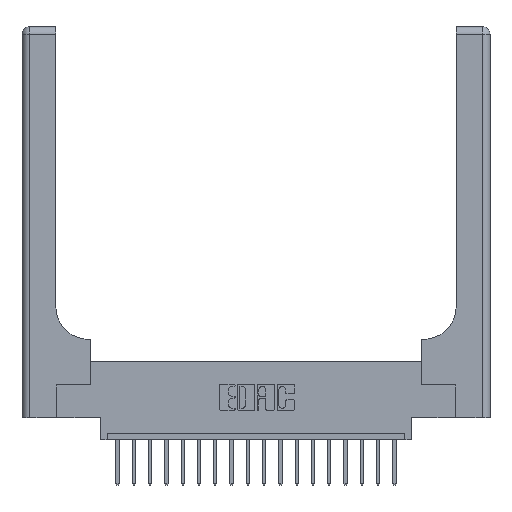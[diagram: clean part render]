
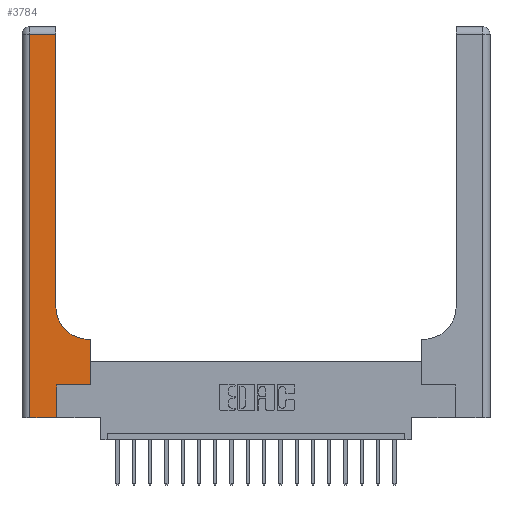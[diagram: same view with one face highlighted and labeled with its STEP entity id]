
A CAD part, top view. The second image highlights one B-rep face of the part: STEP entity #3784.
In plain terms, the highlighted planar face has unit normal (0, 0, 1).
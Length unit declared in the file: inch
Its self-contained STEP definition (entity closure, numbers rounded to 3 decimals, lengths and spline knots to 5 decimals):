
#433 = EDGE_CURVE ( 'NONE', #9430, #5543, #11502, .T. ) ;
#512 = VERTEX_POINT ( 'NONE', #19028 ) ;
#1346 = CARTESIAN_POINT ( 'NONE',  ( 0.26, 2.94, 0.37 ) ) ;
#1496 = PLANE ( 'NONE',  #4193 ) ;
#1530 = ORIENTED_EDGE ( 'NONE', *, *, #11882, .T. ) ;
#1644 = CARTESIAN_POINT ( 'NONE',  ( 0.528, 0.6, 0.37 ) ) ;
#1935 = EDGE_CURVE ( 'NONE', #7485, #10852, #15065, .T. ) ;
#1997 = DIRECTION ( 'NONE',  ( -1., 0., 0. ) ) ;
#2199 = EDGE_CURVE ( 'NONE', #10852, #9343, #11378, .T. ) ;
#2206 = CARTESIAN_POINT ( 'NONE',  ( 0.06, 3., 0.37 ) ) ;
#2723 = CARTESIAN_POINT ( 'NONE',  ( 0.26, 3., 0.37 ) ) ;
#2942 = CIRCLE ( 'NONE', #10118, 0.25 ) ;
#3034 = DIRECTION ( 'NONE',  ( 0., 0., -1. ) ) ;
#3057 = CARTESIAN_POINT ( 'NONE',  ( 0.265, 0., 0.37 ) ) ;
#3190 = ORIENTED_EDGE ( 'NONE', *, *, #14897, .T. ) ;
#3748 = DIRECTION ( 'NONE',  ( 0., 0., -1. ) ) ;
#3783 = EDGE_LOOP ( 'NONE', ( #17732, #6560, #5774, #9302, #17265, #17860, #12624, #1530, #3190 ) ) ;
#3784 = ADVANCED_FACE ( 'NONE', ( #13866 ), #1496, .F. ) ;
#4193 = AXIS2_PLACEMENT_3D ( 'NONE', #4578, #3034, #12538 ) ;
#4578 = CARTESIAN_POINT ( 'NONE',  ( 0., 3., 0.37 ) ) ;
#4712 = VERTEX_POINT ( 'NONE', #10948 ) ;
#5342 = DIRECTION ( 'NONE',  ( 0., 1., 0. ) ) ;
#5543 = VERTEX_POINT ( 'NONE', #14847 ) ;
#5602 = DIRECTION ( 'NONE',  ( 1., 0., 0. ) ) ;
#5774 = ORIENTED_EDGE ( 'NONE', *, *, #12375, .T. ) ;
#5860 = VECTOR ( 'NONE', #15366, 39.37008 ) ;
#6560 = ORIENTED_EDGE ( 'NONE', *, *, #433, .T. ) ;
#7440 = EDGE_CURVE ( 'NONE', #4712, #9430, #12136, .T. ) ;
#7485 = VERTEX_POINT ( 'NONE', #14058 ) ;
#7914 = VERTEX_POINT ( 'NONE', #18507 ) ;
#8312 = CARTESIAN_POINT ( 'NONE',  ( 0., 2.94, 0.37 ) ) ;
#8438 = LINE ( 'NONE', #3057, #14970 ) ;
#8850 = CARTESIAN_POINT ( 'NONE',  ( 0.51, 0.85, 0.37 ) ) ;
#9269 = VERTEX_POINT ( 'NONE', #16557 ) ;
#9302 = ORIENTED_EDGE ( 'NONE', *, *, #16425, .T. ) ;
#9343 = VERTEX_POINT ( 'NONE', #1644 ) ;
#9362 = VECTOR ( 'NONE', #19278, 39.37008 ) ;
#9430 = VERTEX_POINT ( 'NONE', #1346 ) ;
#10118 = AXIS2_PLACEMENT_3D ( 'NONE', #8850, #3748, #5602 ) ;
#10125 = CARTESIAN_POINT ( 'NONE',  ( 0.528, 0.25, 0.37 ) ) ;
#10379 = VECTOR ( 'NONE', #19557, 39.37008 ) ;
#10391 = DIRECTION ( 'NONE',  ( 0., 1., 0. ) ) ;
#10852 = VERTEX_POINT ( 'NONE', #10125 ) ;
#10948 = CARTESIAN_POINT ( 'NONE',  ( 0.26, 0.85, 0.37 ) ) ;
#10988 = DIRECTION ( 'NONE',  ( 1., 0., 0. ) ) ;
#11378 = LINE ( 'NONE', #19315, #14682 ) ;
#11502 = LINE ( 'NONE', #8312, #18469 ) ;
#11882 = EDGE_CURVE ( 'NONE', #9343, #512, #14486, .T. ) ;
#12136 = LINE ( 'NONE', #2723, #15811 ) ;
#12330 = LINE ( 'NONE', #18730, #16670 ) ;
#12375 = EDGE_CURVE ( 'NONE', #5543, #7914, #13345, .T. ) ;
#12538 = DIRECTION ( 'NONE',  ( -1., 0., 0. ) ) ;
#12624 = ORIENTED_EDGE ( 'NONE', *, *, #2199, .T. ) ;
#13345 = LINE ( 'NONE', #2206, #10379 ) ;
#13539 = EDGE_CURVE ( 'NONE', #9269, #7485, #8438, .T. ) ;
#13866 = FACE_OUTER_BOUND ( 'NONE', #3783, .T. ) ;
#14058 = CARTESIAN_POINT ( 'NONE',  ( 0.265, 0.25, 0.37 ) ) ;
#14486 = LINE ( 'NONE', #14587, #9362 ) ;
#14563 = DIRECTION ( 'NONE',  ( 0., 1., 0. ) ) ;
#14587 = CARTESIAN_POINT ( 'NONE',  ( 0.26, 0.6, 0.37 ) ) ;
#14682 = VECTOR ( 'NONE', #5342, 39.37008 ) ;
#14847 = CARTESIAN_POINT ( 'NONE',  ( 0.06, 2.94, 0.37 ) ) ;
#14897 = EDGE_CURVE ( 'NONE', #512, #4712, #2942, .T. ) ;
#14970 = VECTOR ( 'NONE', #14563, 39.37008 ) ;
#15065 = LINE ( 'NONE', #18614, #5860 ) ;
#15366 = DIRECTION ( 'NONE',  ( 1., 0., 0. ) ) ;
#15811 = VECTOR ( 'NONE', #10391, 39.37008 ) ;
#16425 = EDGE_CURVE ( 'NONE', #7914, #9269, #12330, .T. ) ;
#16557 = CARTESIAN_POINT ( 'NONE',  ( 0.265, 0., 0.37 ) ) ;
#16670 = VECTOR ( 'NONE', #10988, 39.37008 ) ;
#17265 = ORIENTED_EDGE ( 'NONE', *, *, #13539, .T. ) ;
#17732 = ORIENTED_EDGE ( 'NONE', *, *, #7440, .T. ) ;
#17860 = ORIENTED_EDGE ( 'NONE', *, *, #1935, .T. ) ;
#18469 = VECTOR ( 'NONE', #1997, 39.37008 ) ;
#18507 = CARTESIAN_POINT ( 'NONE',  ( 0.06, 0., 0.37 ) ) ;
#18614 = CARTESIAN_POINT ( 'NONE',  ( 0.265, 0.25, 0.37 ) ) ;
#18730 = CARTESIAN_POINT ( 'NONE',  ( 0., 0., 0.37 ) ) ;
#19028 = CARTESIAN_POINT ( 'NONE',  ( 0.51, 0.6, 0.37 ) ) ;
#19278 = DIRECTION ( 'NONE',  ( -1., 0., 0. ) ) ;
#19315 = CARTESIAN_POINT ( 'NONE',  ( 0.528, 0.25, 0.37 ) ) ;
#19557 = DIRECTION ( 'NONE',  ( 0., -1., 0. ) ) ;
